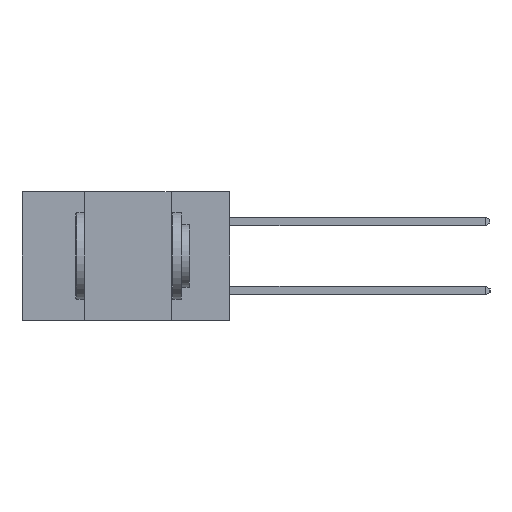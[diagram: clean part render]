
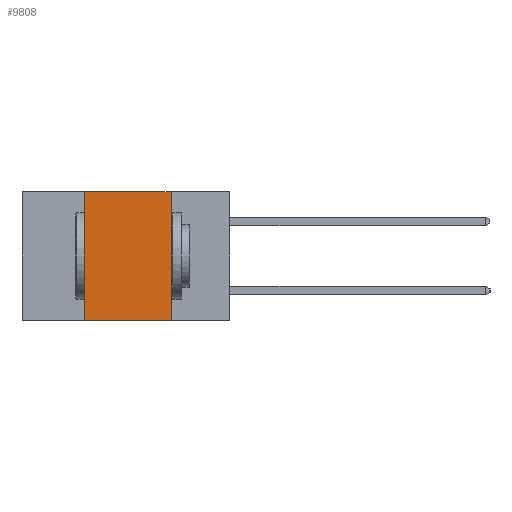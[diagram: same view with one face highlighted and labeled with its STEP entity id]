
A CAD part, left-side view. The second image highlights one B-rep face of the part: STEP entity #9808.
In plain terms, the highlighted planar face has unit normal (-1, 0, 0).
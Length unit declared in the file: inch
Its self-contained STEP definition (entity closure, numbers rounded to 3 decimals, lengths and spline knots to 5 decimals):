
#505 = VERTEX_POINT ( 'NONE', #3902 ) ;
#1454 = CARTESIAN_POINT ( 'NONE',  ( 0., 0.6, -0.37 ) ) ;
#1464 = DIRECTION ( 'NONE',  ( 0., -1., 0. ) ) ;
#2195 = VECTOR ( 'NONE', #10080, 39.37008 ) ;
#2356 = EDGE_CURVE ( 'NONE', #2966, #10800, #11153, .T. ) ;
#2892 = CARTESIAN_POINT ( 'NONE',  ( 0., 0.17, 0. ) ) ;
#2917 = ORIENTED_EDGE ( 'NONE', *, *, #4628, .T. ) ;
#2966 = VERTEX_POINT ( 'NONE', #12415 ) ;
#3128 = CARTESIAN_POINT ( 'NONE',  ( 0., 0.6, 0. ) ) ;
#3583 = ORIENTED_EDGE ( 'NONE', *, *, #5066, .F. ) ;
#3757 = AXIS2_PLACEMENT_3D ( 'NONE', #7882, #7420, #7368 ) ;
#3902 = CARTESIAN_POINT ( 'NONE',  ( 0., 0.42, -0.37 ) ) ;
#4141 = EDGE_LOOP ( 'NONE', ( #3583, #10752, #8226, #2917 ) ) ;
#4628 = EDGE_CURVE ( 'NONE', #505, #5817, #7527, .T. ) ;
#4891 = VECTOR ( 'NONE', #1464, 39.37008 ) ;
#5066 = EDGE_CURVE ( 'NONE', #10800, #5817, #7841, .T. ) ;
#5817 = VERTEX_POINT ( 'NONE', #9435 ) ;
#7368 = DIRECTION ( 'NONE',  ( 0., 0., -1. ) ) ;
#7420 = DIRECTION ( 'NONE',  ( 1., 0., 0. ) ) ;
#7527 = LINE ( 'NONE', #1454, #4891 ) ;
#7533 = PLANE ( 'NONE',  #3757 ) ;
#7841 = LINE ( 'NONE', #9963, #2195 ) ;
#7882 = CARTESIAN_POINT ( 'NONE',  ( 0., 0.6, 0. ) ) ;
#7903 = VECTOR ( 'NONE', #9900, 39.37008 ) ;
#7957 = EDGE_CURVE ( 'NONE', #505, #2966, #10447, .T. ) ;
#8226 = ORIENTED_EDGE ( 'NONE', *, *, #7957, .F. ) ;
#8482 = CARTESIAN_POINT ( 'NONE',  ( 0., 0.42, -0.37 ) ) ;
#8950 = VECTOR ( 'NONE', #9777, 39.37008 ) ;
#9435 = CARTESIAN_POINT ( 'NONE',  ( 0., 0.17, -0.37 ) ) ;
#9777 = DIRECTION ( 'NONE',  ( 0., -1., 0. ) ) ;
#9808 = ADVANCED_FACE ( 'NONE', ( #10413 ), #7533, .F. ) ;
#9900 = DIRECTION ( 'NONE',  ( 0., 0., 1. ) ) ;
#9963 = CARTESIAN_POINT ( 'NONE',  ( 0., 0.17, -0.37 ) ) ;
#10080 = DIRECTION ( 'NONE',  ( 0., 0., -1. ) ) ;
#10413 = FACE_OUTER_BOUND ( 'NONE', #4141, .T. ) ;
#10447 = LINE ( 'NONE', #8482, #7903 ) ;
#10752 = ORIENTED_EDGE ( 'NONE', *, *, #2356, .F. ) ;
#10800 = VERTEX_POINT ( 'NONE', #2892 ) ;
#11153 = LINE ( 'NONE', #3128, #8950 ) ;
#12415 = CARTESIAN_POINT ( 'NONE',  ( 0., 0.42, 0. ) ) ;
